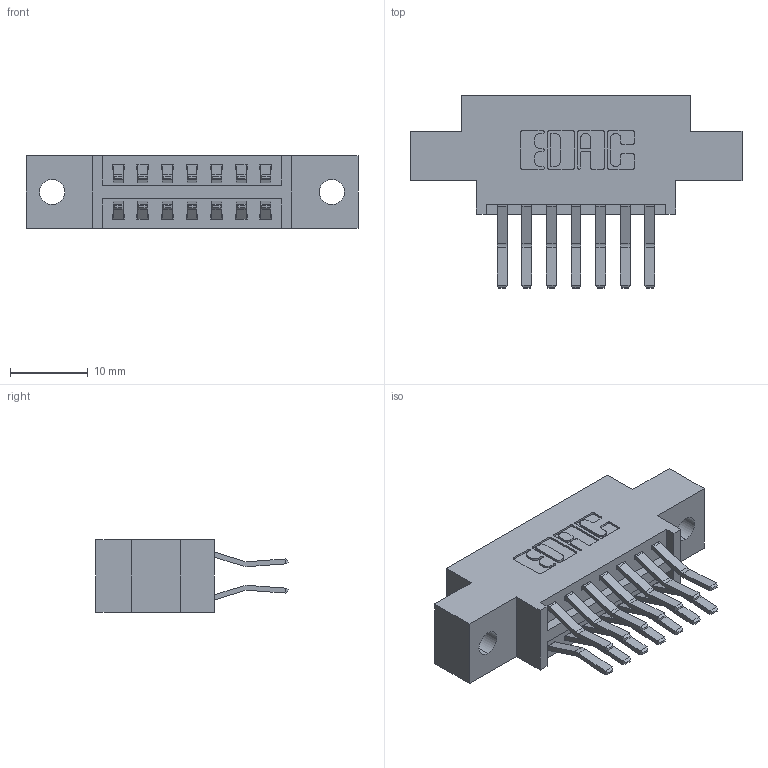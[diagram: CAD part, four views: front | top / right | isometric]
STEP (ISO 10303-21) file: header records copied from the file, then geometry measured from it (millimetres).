
FILE_DESCRIPTION (( 'STEP AP203' ), '1' );
FILE_NAME ('396-014-560-802.STEP', '2019-11-01T17:25:00', ( '' ), ( '' ), 'SwSTEP 2.0', 'SolidWorks 2016', '' );
FILE_SCHEMA (( 'CONFIG_CONTROL_DESIGN' ));
Length unit declared in the file: inch
Products named in the file (3): 345-292-001_560 Tail; 396-014-560-802; 346 Part_0.170 Offset - 0.128 Dia
Assembly tree (15 placements, depth 2):
  396-014-560-802
    346 Part_0.170 Offset - 0.128 Dia
    345-292-001_560 Tail  x14
Bounding box: 42.8 x 24.78 x 9.4 mm (x, y, z)
Volume: 3802.1 mm3; surface area: 4831.3 mm2
Topology: 15 solids, 15 shells, 882 faces, 2595 edges, 1710 vertices
Faces by surface type: plane 570, cylinder 312
Entity records: 9503 total; most frequent: CARTESIAN_POINT 1616, ORIENTED_EDGE 1550, DIRECTION 1479, EDGE_CURVE 775, LINE 611, VECTOR 611, VERTEX_POINT 514, AXIS2_PLACEMENT_3D 434
